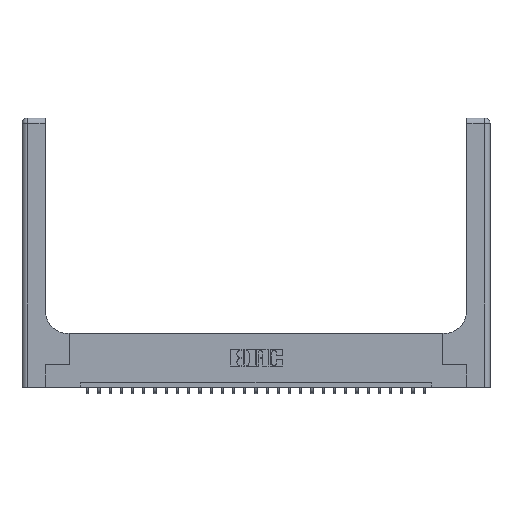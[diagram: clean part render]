
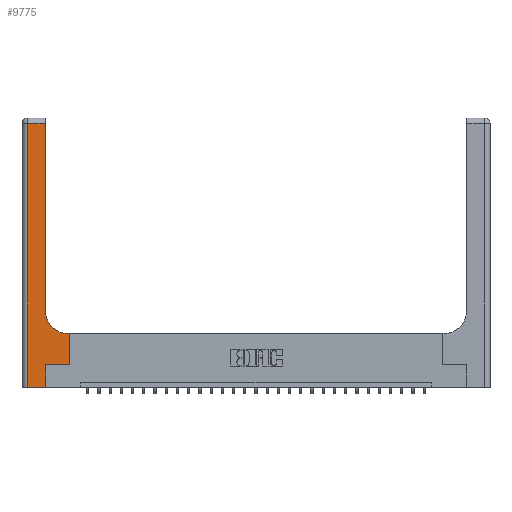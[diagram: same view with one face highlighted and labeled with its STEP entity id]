
A CAD part, top view. The second image highlights one B-rep face of the part: STEP entity #9775.
In plain terms, the highlighted planar face has unit normal (0, 0, 1).
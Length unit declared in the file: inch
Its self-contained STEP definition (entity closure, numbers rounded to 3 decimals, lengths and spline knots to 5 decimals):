
#40 = CARTESIAN_POINT ( 'NONE',  ( 0., 2.94, 0.37 ) ) ;
#316 = VERTEX_POINT ( 'NONE', #14889 ) ;
#321 = CARTESIAN_POINT ( 'NONE',  ( 0.265, 0.25, 0.37 ) ) ;
#1094 = EDGE_CURVE ( 'NONE', #24771, #24260, #23093, .T. ) ;
#1179 = ORIENTED_EDGE ( 'NONE', *, *, #1094, .T. ) ;
#1834 = EDGE_CURVE ( 'NONE', #8375, #3501, #18338, .T. ) ;
#2303 = DIRECTION ( 'NONE',  ( 1., 0., 0. ) ) ;
#2413 = ORIENTED_EDGE ( 'NONE', *, *, #11950, .T. ) ;
#2431 = EDGE_CURVE ( 'NONE', #316, #12164, #18499, .T. ) ;
#2976 = FACE_OUTER_BOUND ( 'NONE', #24667, .T. ) ;
#3255 = ORIENTED_EDGE ( 'NONE', *, *, #6361, .T. ) ;
#3501 = VERTEX_POINT ( 'NONE', #15091 ) ;
#4340 = CARTESIAN_POINT ( 'NONE',  ( 0.265, 0.25, 0.37 ) ) ;
#4657 = ORIENTED_EDGE ( 'NONE', *, *, #7320, .T. ) ;
#4982 = DIRECTION ( 'NONE',  ( -1., 0., 0. ) ) ;
#5135 = CARTESIAN_POINT ( 'NONE',  ( 0.06, 0., 0.37 ) ) ;
#5202 = CARTESIAN_POINT ( 'NONE',  ( 0.26, 0.6, 0.37 ) ) ;
#6361 = EDGE_CURVE ( 'NONE', #18380, #23285, #21182, .T. ) ;
#6504 = EDGE_CURVE ( 'NONE', #24260, #18746, #15023, .T. ) ;
#6917 = VECTOR ( 'NONE', #23711, 39.37008 ) ;
#6945 = VECTOR ( 'NONE', #16317, 39.37008 ) ;
#7061 = LINE ( 'NONE', #5202, #25615 ) ;
#7320 = EDGE_CURVE ( 'NONE', #23285, #316, #7061, .T. ) ;
#7943 = DIRECTION ( 'NONE',  ( 0., -1., 0. ) ) ;
#8005 = ORIENTED_EDGE ( 'NONE', *, *, #6504, .T. ) ;
#8072 = ORIENTED_EDGE ( 'NONE', *, *, #2431, .T. ) ;
#8375 = VERTEX_POINT ( 'NONE', #13135 ) ;
#8384 = AXIS2_PLACEMENT_3D ( 'NONE', #20781, #11138, #4982 ) ;
#9449 = CARTESIAN_POINT ( 'NONE',  ( 0.06, 3., 0.37 ) ) ;
#9583 = LINE ( 'NONE', #9449, #24714 ) ;
#9775 = ADVANCED_FACE ( 'NONE', ( #2976 ), #25312, .F. ) ;
#10022 = ORIENTED_EDGE ( 'NONE', *, *, #16443, .T. ) ;
#10849 = CARTESIAN_POINT ( 'NONE',  ( 0.528, 0.6, 0.37 ) ) ;
#11138 = DIRECTION ( 'NONE',  ( 0., 0., -1. ) ) ;
#11385 = VECTOR ( 'NONE', #2303, 39.37008 ) ;
#11484 = ORIENTED_EDGE ( 'NONE', *, *, #21612, .T. ) ;
#11950 = EDGE_CURVE ( 'NONE', #3501, #24771, #9583, .T. ) ;
#12164 = VERTEX_POINT ( 'NONE', #21209 ) ;
#12605 = CARTESIAN_POINT ( 'NONE',  ( 0.528, 0.25, 0.37 ) ) ;
#13135 = CARTESIAN_POINT ( 'NONE',  ( 0.26, 2.94, 0.37 ) ) ;
#14565 = DIRECTION ( 'NONE',  ( 0., 0., -1. ) ) ;
#14889 = CARTESIAN_POINT ( 'NONE',  ( 0.51, 0.6, 0.37 ) ) ;
#15023 = LINE ( 'NONE', #16620, #21713 ) ;
#15058 = CARTESIAN_POINT ( 'NONE',  ( 0., 0., 0.37 ) ) ;
#15091 = CARTESIAN_POINT ( 'NONE',  ( 0.06, 2.94, 0.37 ) ) ;
#15522 = AXIS2_PLACEMENT_3D ( 'NONE', #20730, #14565, #22452 ) ;
#16317 = DIRECTION ( 'NONE',  ( -1., 0., 0. ) ) ;
#16443 = EDGE_CURVE ( 'NONE', #12164, #8375, #25733, .T. ) ;
#16620 = CARTESIAN_POINT ( 'NONE',  ( 0.265, 0., 0.37 ) ) ;
#16729 = ORIENTED_EDGE ( 'NONE', *, *, #1834, .T. ) ;
#16970 = CARTESIAN_POINT ( 'NONE',  ( 0.528, 0.25, 0.37 ) ) ;
#17146 = VECTOR ( 'NONE', #23348, 39.37008 ) ;
#18338 = LINE ( 'NONE', #40, #6945 ) ;
#18380 = VERTEX_POINT ( 'NONE', #16970 ) ;
#18499 = CIRCLE ( 'NONE', #15522, 0.25 ) ;
#18746 = VERTEX_POINT ( 'NONE', #4340 ) ;
#19580 = CARTESIAN_POINT ( 'NONE',  ( 0.26, 3., 0.37 ) ) ;
#20730 = CARTESIAN_POINT ( 'NONE',  ( 0.51, 0.85, 0.37 ) ) ;
#20781 = CARTESIAN_POINT ( 'NONE',  ( 0., 3., 0.37 ) ) ;
#20904 = LINE ( 'NONE', #321, #11385 ) ;
#21182 = LINE ( 'NONE', #12605, #23823 ) ;
#21209 = CARTESIAN_POINT ( 'NONE',  ( 0.26, 0.85, 0.37 ) ) ;
#21371 = CARTESIAN_POINT ( 'NONE',  ( 0.265, 0., 0.37 ) ) ;
#21612 = EDGE_CURVE ( 'NONE', #18746, #18380, #20904, .T. ) ;
#21713 = VECTOR ( 'NONE', #24784, 39.37008 ) ;
#22452 = DIRECTION ( 'NONE',  ( 1., 0., 0. ) ) ;
#22913 = DIRECTION ( 'NONE',  ( 0., 1., 0. ) ) ;
#23093 = LINE ( 'NONE', #15058, #17146 ) ;
#23285 = VERTEX_POINT ( 'NONE', #10849 ) ;
#23348 = DIRECTION ( 'NONE',  ( 1., 0., 0. ) ) ;
#23518 = DIRECTION ( 'NONE',  ( -1., 0., 0. ) ) ;
#23711 = DIRECTION ( 'NONE',  ( 0., 1., 0. ) ) ;
#23823 = VECTOR ( 'NONE', #22913, 39.37008 ) ;
#24260 = VERTEX_POINT ( 'NONE', #21371 ) ;
#24667 = EDGE_LOOP ( 'NONE', ( #10022, #16729, #2413, #1179, #8005, #11484, #3255, #4657, #8072 ) ) ;
#24714 = VECTOR ( 'NONE', #7943, 39.37008 ) ;
#24771 = VERTEX_POINT ( 'NONE', #5135 ) ;
#24784 = DIRECTION ( 'NONE',  ( 0., 1., 0. ) ) ;
#25312 = PLANE ( 'NONE',  #8384 ) ;
#25615 = VECTOR ( 'NONE', #23518, 39.37008 ) ;
#25733 = LINE ( 'NONE', #19580, #6917 ) ;
